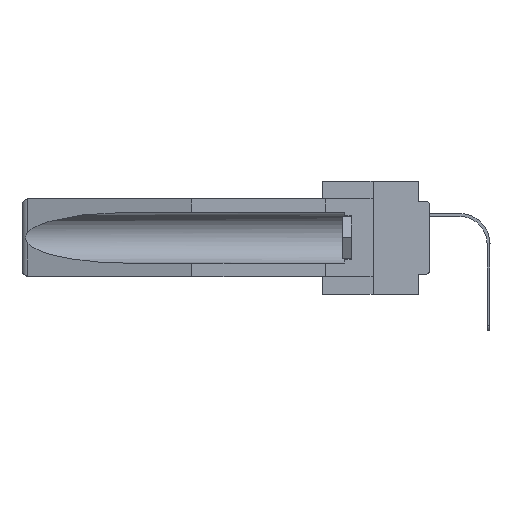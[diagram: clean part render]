
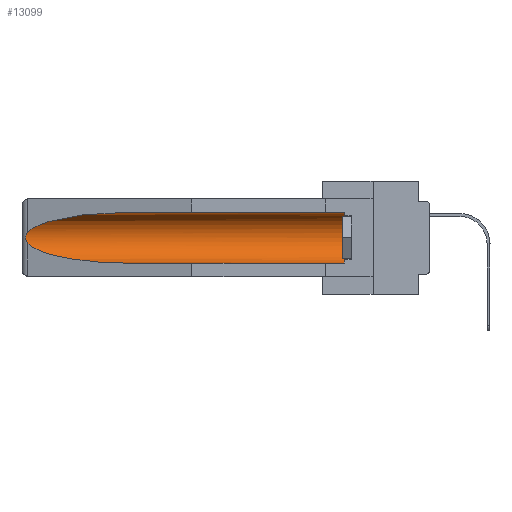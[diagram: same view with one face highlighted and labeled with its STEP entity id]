
A CAD part, left-side view. The second image highlights one B-rep face of the part: STEP entity #13099.
In plain terms, the highlighted cylindrical face has radius 2.857 mm (diameter 5.715 mm), a partial arc.
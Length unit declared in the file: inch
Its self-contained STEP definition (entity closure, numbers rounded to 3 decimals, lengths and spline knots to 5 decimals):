
#313 = CIRCLE ( 'NONE', #17099, 0.1125 ) ;
#676 = CARTESIAN_POINT ( 'NONE',  ( 0.26537, 1.52718, -0.19328 ) ) ;
#2991 = EDGE_CURVE ( 'NONE', #17465, #27002, #28168, .T. ) ;
#4648 = ORIENTED_EDGE ( 'NONE', *, *, #36430, .T. ) ;
#4968 = LINE ( 'NONE', #31416, #18619 ) ;
#6930 = DIRECTION ( 'NONE',  ( 0., 1., 0. ) ) ;
#8627 = ORIENTED_EDGE ( 'NONE', *, *, #28062, .T. ) ;
#9142 = EDGE_CURVE ( 'NONE', #27002, #33328, #18900, .T. ) ;
#9276 = CARTESIAN_POINT ( 'NONE',  ( 0.25451, 1.48313, -0.24835 ) ) ;
#10034 = DIRECTION ( 'NONE',  ( 0., -1., 0. ) ) ;
#11295 = CARTESIAN_POINT ( 'NONE',  ( 0.26537, 1.52718, -0.14972 ) ) ;
#11764 = CARTESIAN_POINT ( 'NONE',  ( 0.2675, 1.53308, -0.16763 ) ) ;
#12221 = CARTESIAN_POINT ( 'NONE',  ( 0.155, 1.07973, -0.059 ) ) ;
#12250 = CARTESIAN_POINT ( 'NONE',  ( 0.155, 1.07973, -0.059 ) ) ;
#12847 = CARTESIAN_POINT ( 'NONE',  ( 0.155, 1.07973, -0.284 ) ) ;
#13099 = ADVANCED_FACE ( 'NONE', ( #20154 ), #17338, .F. ) ;
#13600 = DIRECTION ( 'NONE',  ( 0., 1., 0. ) ) ;
#14750 = CARTESIAN_POINT ( 'NONE',  ( 0.26537, 1.52718, -0.14972 ) ) ;
#15211 = CARTESIAN_POINT ( 'NONE',  ( 0.26537, 1.52718, -0.14972 ) ) ;
#15550 = LINE ( 'NONE', #24190, #35232 ) ;
#15840 = DIRECTION ( 'NONE',  ( 0., 0., 1. ) ) ;
#17099 = AXIS2_PLACEMENT_3D ( 'NONE', #30480, #10034, #15840 ) ;
#17338 = CYLINDRICAL_SURFACE ( 'NONE', #19967, 0.1125 ) ;
#17465 = VERTEX_POINT ( 'NONE', #11295 ) ;
#17534 = CARTESIAN_POINT ( 'NONE',  ( 0.21114, 1.30732, -0.284 ) ) ;
#17715 = CARTESIAN_POINT ( 'NONE',  ( 0.26537, 1.52718, -0.19328 ) ) ;
#18619 = VECTOR ( 'NONE', #13600, 39.37008 ) ;
#18808 = EDGE_CURVE ( 'NONE', #29616, #17465, #21085, .T. ) ;
#18900 =( BOUNDED_CURVE ( )  B_SPLINE_CURVE ( 3, ( #17715, #9276, #17534, #20709 ),
 .UNSPECIFIED., .F., .F. ) 
 B_SPLINE_CURVE_WITH_KNOTS ( ( 4, 4 ),
 ( 0.1948, 1.5708 ),
 .UNSPECIFIED. ) 
 CURVE ( )  GEOMETRIC_REPRESENTATION_ITEM ( )  RATIONAL_B_SPLINE_CURVE ( ( 1., 0.848, 0.848, 1. ) ) 
 REPRESENTATION_ITEM ( '' )  );
#19781 = CARTESIAN_POINT ( 'NONE',  ( 0.26537, 1.52718, -0.19328 ) ) ;
#19825 = CARTESIAN_POINT ( 'NONE',  ( 0.26597, 1.52961, -0.15275 ) ) ;
#19967 = AXIS2_PLACEMENT_3D ( 'NONE', #31789, #28986, #34051 ) ;
#20154 = FACE_OUTER_BOUND ( 'NONE', #22997, .T. ) ;
#20709 = CARTESIAN_POINT ( 'NONE',  ( 0.155, 1.07973, -0.284 ) ) ;
#21085 =( BOUNDED_CURVE ( )  B_SPLINE_CURVE ( 3, ( #12221, #23293, #23665, #15211 ),
 .UNSPECIFIED., .F., .F. ) 
 B_SPLINE_CURVE_WITH_KNOTS ( ( 4, 4 ),
 ( 4.71239, 6.08839 ),
 .UNSPECIFIED. ) 
 CURVE ( )  GEOMETRIC_REPRESENTATION_ITEM ( )  RATIONAL_B_SPLINE_CURVE ( ( 1., 0.848, 0.848, 1. ) ) 
 REPRESENTATION_ITEM ( '' )  );
#22963 = CARTESIAN_POINT ( 'NONE',  ( 0.155, 0.126, -0.284 ) ) ;
#22997 = EDGE_LOOP ( 'NONE', ( #30238, #32401, #24337, #25190, #8627, #4648 ) ) ;
#23018 = CARTESIAN_POINT ( 'NONE',  ( 0.26654, 1.53092, -0.15636 ) ) ;
#23293 = CARTESIAN_POINT ( 'NONE',  ( 0.21114, 1.30732, -0.059 ) ) ;
#23401 = VERTEX_POINT ( 'NONE', #22963 ) ;
#23665 = CARTESIAN_POINT ( 'NONE',  ( 0.25451, 1.48313, -0.09465 ) ) ;
#24190 = CARTESIAN_POINT ( 'NONE',  ( 0.155, -0.30754, -0.284 ) ) ;
#24337 = ORIENTED_EDGE ( 'NONE', *, *, #9142, .T. ) ;
#25190 = ORIENTED_EDGE ( 'NONE', *, *, #32404, .F. ) ;
#26017 = CARTESIAN_POINT ( 'NONE',  ( 0.2673, 1.53269, -0.17917 ) ) ;
#26385 = CARTESIAN_POINT ( 'NONE',  ( 0.26655, 1.53094, -0.18657 ) ) ;
#27002 = VERTEX_POINT ( 'NONE', #19781 ) ;
#28062 = EDGE_CURVE ( 'NONE', #23401, #35661, #313, .T. ) ;
#28168 = B_SPLINE_CURVE_WITH_KNOTS ( 'NONE', 3,
 ( #14750, #19825, #23018, #37099, #11764, #31833, #26017, #26385, #31286, #676 ),
 .UNSPECIFIED., .F., .F.,
 ( 4, 2, 2, 2, 4 ),
 ( 0., 0.00029, 0.00058, 0.00087, 0.00117 ),
 .UNSPECIFIED. ) ;
#28986 = DIRECTION ( 'NONE',  ( 0., 1., 0. ) ) ;
#29616 = VERTEX_POINT ( 'NONE', #12250 ) ;
#30238 = ORIENTED_EDGE ( 'NONE', *, *, #18808, .T. ) ;
#30480 = CARTESIAN_POINT ( 'NONE',  ( 0.155, 0.126, -0.1715 ) ) ;
#31286 = CARTESIAN_POINT ( 'NONE',  ( 0.26597, 1.5296, -0.19026 ) ) ;
#31416 = CARTESIAN_POINT ( 'NONE',  ( 0.155, -0.30754, -0.059 ) ) ;
#31789 = CARTESIAN_POINT ( 'NONE',  ( 0.155, -0.30754, -0.1715 ) ) ;
#31833 = CARTESIAN_POINT ( 'NONE',  ( 0.2675, 1.53308, -0.17534 ) ) ;
#32375 = CARTESIAN_POINT ( 'NONE',  ( 0.155, 0.126, -0.059 ) ) ;
#32401 = ORIENTED_EDGE ( 'NONE', *, *, #2991, .T. ) ;
#32404 = EDGE_CURVE ( 'NONE', #23401, #33328, #15550, .T. ) ;
#33328 = VERTEX_POINT ( 'NONE', #12847 ) ;
#34051 = DIRECTION ( 'NONE',  ( 0., 0., 1. ) ) ;
#35232 = VECTOR ( 'NONE', #6930, 39.37008 ) ;
#35661 = VERTEX_POINT ( 'NONE', #32375 ) ;
#36430 = EDGE_CURVE ( 'NONE', #35661, #29616, #4968, .T. ) ;
#37099 = CARTESIAN_POINT ( 'NONE',  ( 0.2673, 1.5327, -0.16383 ) ) ;
